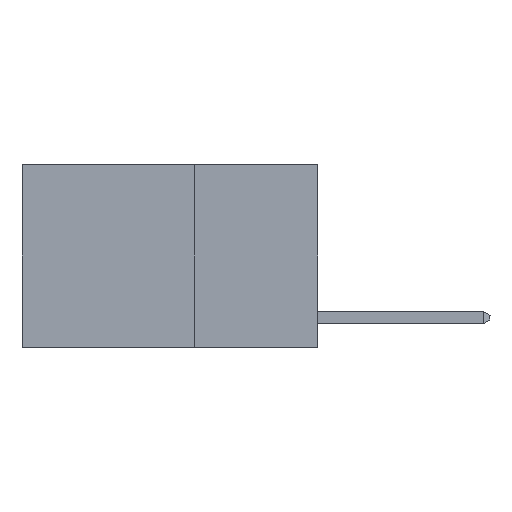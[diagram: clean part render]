
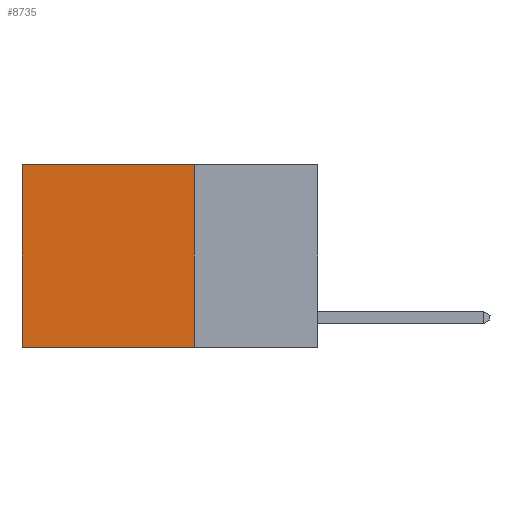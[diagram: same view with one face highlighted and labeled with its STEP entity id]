
A CAD part, left-side view. The second image highlights one B-rep face of the part: STEP entity #8735.
In plain terms, the highlighted planar face has unit normal (-1, 0, 0).
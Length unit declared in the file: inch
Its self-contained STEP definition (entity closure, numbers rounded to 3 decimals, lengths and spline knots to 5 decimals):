
#169 = AXIS2_PLACEMENT_3D ( 'NONE', #6245, #302, #2490 ) ;
#302 = DIRECTION ( 'NONE',  ( 1., 0., 0. ) ) ;
#345 = FACE_OUTER_BOUND ( 'NONE', #408, .T. ) ;
#408 = EDGE_LOOP ( 'NONE', ( #1840, #4958, #8914, #4638 ) ) ;
#1098 = VECTOR ( 'NONE', #1935, 39.37008 ) ;
#1600 = VECTOR ( 'NONE', #4247, 39.37008 ) ;
#1840 = ORIENTED_EDGE ( 'NONE', *, *, #8769, .T. ) ;
#1935 = DIRECTION ( 'NONE',  ( 0., 0., -1. ) ) ;
#2490 = DIRECTION ( 'NONE',  ( 0., 0., -1. ) ) ;
#2700 = LINE ( 'NONE', #8689, #1098 ) ;
#2791 = VECTOR ( 'NONE', #8833, 39.37008 ) ;
#3326 = VERTEX_POINT ( 'NONE', #8154 ) ;
#3464 = VERTEX_POINT ( 'NONE', #6141 ) ;
#4247 = DIRECTION ( 'NONE',  ( 0., 0., -1. ) ) ;
#4433 = VECTOR ( 'NONE', #8688, 39.37008 ) ;
#4638 = ORIENTED_EDGE ( 'NONE', *, *, #7028, .T. ) ;
#4657 = CARTESIAN_POINT ( 'NONE',  ( 0.2625, 0.25, -0.37 ) ) ;
#4782 = PLANE ( 'NONE',  #169 ) ;
#4840 = VERTEX_POINT ( 'NONE', #9551 ) ;
#4936 = CARTESIAN_POINT ( 'NONE',  ( 0.2625, 0.6, 0. ) ) ;
#4958 = ORIENTED_EDGE ( 'NONE', *, *, #8483, .F. ) ;
#4998 = CARTESIAN_POINT ( 'NONE',  ( 0.2625, 0.25, 0. ) ) ;
#5342 = EDGE_CURVE ( 'NONE', #4840, #3464, #8703, .T. ) ;
#6131 = LINE ( 'NONE', #4657, #2791 ) ;
#6141 = CARTESIAN_POINT ( 'NONE',  ( 0.2625, 0.25, -0.37 ) ) ;
#6245 = CARTESIAN_POINT ( 'NONE',  ( 0.2625, 0.25, 0. ) ) ;
#6541 = CARTESIAN_POINT ( 'NONE',  ( 0.2625, 0.25, 0. ) ) ;
#7023 = VERTEX_POINT ( 'NONE', #4936 ) ;
#7028 = EDGE_CURVE ( 'NONE', #4840, #7023, #7938, .T. ) ;
#7938 = LINE ( 'NONE', #6541, #4433 ) ;
#8154 = CARTESIAN_POINT ( 'NONE',  ( 0.2625, 0.6, -0.37 ) ) ;
#8483 = EDGE_CURVE ( 'NONE', #3464, #3326, #6131, .T. ) ;
#8688 = DIRECTION ( 'NONE',  ( 0., 1., 0. ) ) ;
#8689 = CARTESIAN_POINT ( 'NONE',  ( 0.2625, 0.6, 0. ) ) ;
#8703 = LINE ( 'NONE', #4998, #1600 ) ;
#8735 = ADVANCED_FACE ( 'NONE', ( #345 ), #4782, .F. ) ;
#8769 = EDGE_CURVE ( 'NONE', #7023, #3326, #2700, .T. ) ;
#8833 = DIRECTION ( 'NONE',  ( 0., 1., 0. ) ) ;
#8914 = ORIENTED_EDGE ( 'NONE', *, *, #5342, .F. ) ;
#9551 = CARTESIAN_POINT ( 'NONE',  ( 0.2625, 0.25, 0. ) ) ;
